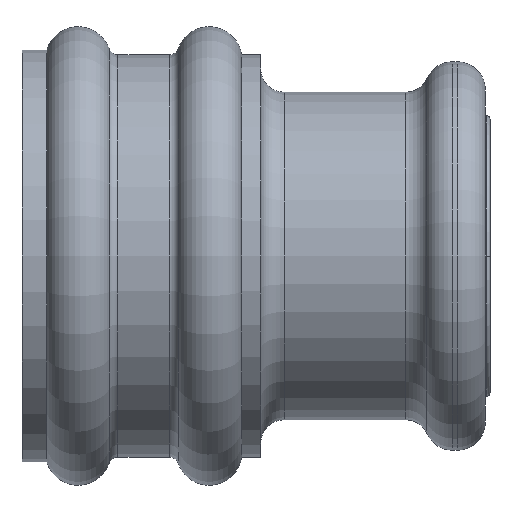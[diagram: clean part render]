
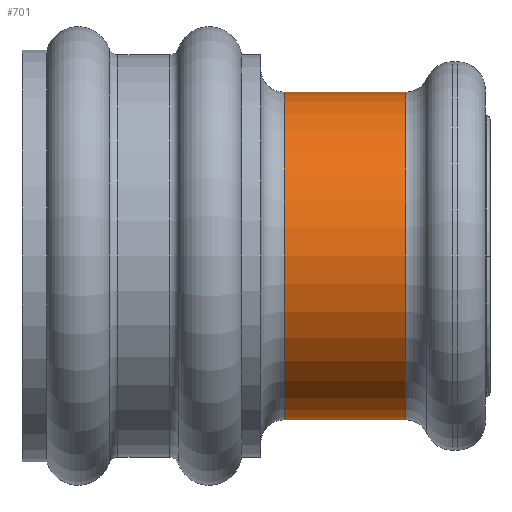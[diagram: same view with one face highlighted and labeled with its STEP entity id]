
A CAD part, left-side view. The second image highlights one B-rep face of the part: STEP entity #701.
In plain terms, the highlighted cylindrical face has radius 1.75 mm (diameter 3.5 mm), a partial arc.
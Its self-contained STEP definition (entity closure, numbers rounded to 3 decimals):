
#30 = CARTESIAN_POINT ( 'NONE',  ( 0., 31.902, 0.4 ) ) ;
#61 = DIRECTION ( 'NONE',  ( 0., 1., 0. ) ) ;
#75 = CARTESIAN_POINT ( 'NONE',  ( 0., 31.902, -3.1 ) ) ;
#79 = DIRECTION ( 'NONE',  ( 0., 0., -1. ) ) ;
#147 = VECTOR ( 'NONE', #815, 1000. ) ;
#150 = ORIENTED_EDGE ( 'NONE', *, *, #971, .T. ) ;
#243 = CARTESIAN_POINT ( 'NONE',  ( 0., 33.2, 0.4 ) ) ;
#263 = EDGE_CURVE ( 'NONE', #1367, #517, #668, .T. ) ;
#270 = CIRCLE ( 'NONE', #596, 1.75 ) ;
#275 = DIRECTION ( 'NONE',  ( 0., -1., 0. ) ) ;
#390 = AXIS2_PLACEMENT_3D ( 'NONE', #822, #275, #548 ) ;
#464 = DIRECTION ( 'NONE',  ( 0., 0., 1. ) ) ;
#517 = VERTEX_POINT ( 'NONE', #531 ) ;
#531 = CARTESIAN_POINT ( 'NONE',  ( 0., 33.2, -3.1 ) ) ;
#548 = DIRECTION ( 'NONE',  ( 0., 0., 1. ) ) ;
#569 = CYLINDRICAL_SURFACE ( 'NONE', #706, 1.75 ) ;
#588 = DIRECTION ( 'NONE',  ( 0., -1., 0. ) ) ;
#596 = AXIS2_PLACEMENT_3D ( 'NONE', #1260, #588, #464 ) ;
#649 = ORIENTED_EDGE ( 'NONE', *, *, #1607, .F. ) ;
#668 = LINE ( 'NONE', #1213, #147 ) ;
#701 = ADVANCED_FACE ( 'NONE', ( #1144 ), #569, .T. ) ;
#706 = AXIS2_PLACEMENT_3D ( 'NONE', #1282, #995, #79 ) ;
#779 = EDGE_CURVE ( 'NONE', #1511, #517, #270, .T. ) ;
#815 = DIRECTION ( 'NONE',  ( 0., 1., 0. ) ) ;
#822 = CARTESIAN_POINT ( 'NONE',  ( 0., 31.902, -1.35 ) ) ;
#851 = ORIENTED_EDGE ( 'NONE', *, *, #779, .T. ) ;
#858 = EDGE_LOOP ( 'NONE', ( #987, #649, #150, #851 ) ) ;
#879 = CIRCLE ( 'NONE', #390, 1.75 ) ;
#971 = EDGE_CURVE ( 'NONE', #1103, #1511, #1258, .T. ) ;
#987 = ORIENTED_EDGE ( 'NONE', *, *, #263, .F. ) ;
#995 = DIRECTION ( 'NONE',  ( 0., 1., 0. ) ) ;
#1103 = VERTEX_POINT ( 'NONE', #30 ) ;
#1144 = FACE_OUTER_BOUND ( 'NONE', #858, .T. ) ;
#1213 = CARTESIAN_POINT ( 'NONE',  ( 0., 31.902, -3.1 ) ) ;
#1258 = LINE ( 'NONE', #1268, #1666 ) ;
#1260 = CARTESIAN_POINT ( 'NONE',  ( 0., 33.2, -1.35 ) ) ;
#1268 = CARTESIAN_POINT ( 'NONE',  ( 0., 31.902, 0.4 ) ) ;
#1282 = CARTESIAN_POINT ( 'NONE',  ( 0., 30.75, -1.35 ) ) ;
#1367 = VERTEX_POINT ( 'NONE', #75 ) ;
#1511 = VERTEX_POINT ( 'NONE', #243 ) ;
#1607 = EDGE_CURVE ( 'NONE', #1103, #1367, #879, .T. ) ;
#1666 = VECTOR ( 'NONE', #61, 1000. ) ;
